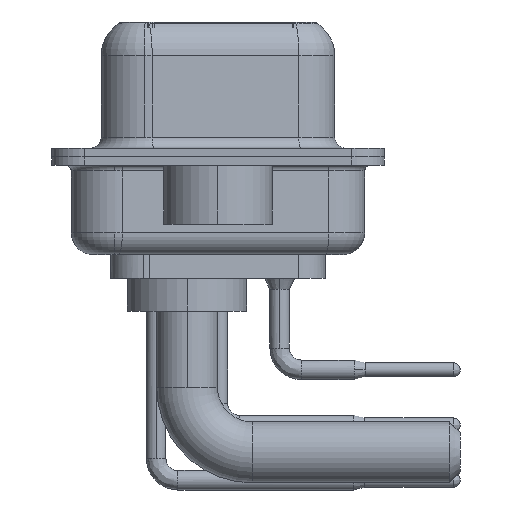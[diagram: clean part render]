
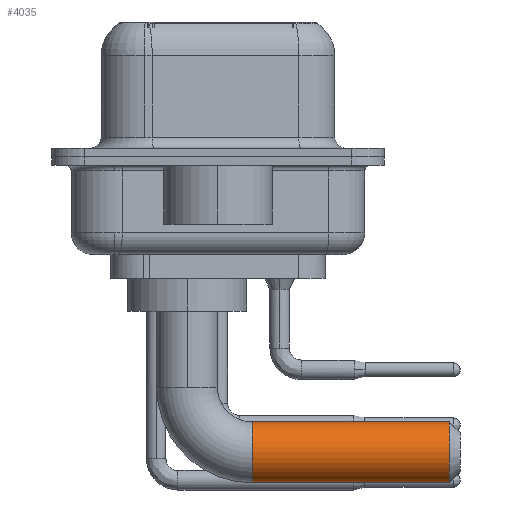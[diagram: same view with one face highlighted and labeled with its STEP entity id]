
A CAD part, left-side view. The second image highlights one B-rep face of the part: STEP entity #4035.
In plain terms, the highlighted cylindrical face has radius 1.4 mm (diameter 2.8 mm), a partial arc.
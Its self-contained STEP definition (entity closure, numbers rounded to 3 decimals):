
#2167 = CIRCLE ( 'NONE', #16886, 1.4 ) ;
#2221 = CARTESIAN_POINT ( 'NONE',  ( 0., -3., -5.1 ) ) ;
#2229 = CARTESIAN_POINT ( 'NONE',  ( 0., -3., -5.1 ) ) ;
#2546 = ORIENTED_EDGE ( 'NONE', *, *, #19837, .F. ) ;
#2560 = VECTOR ( 'NONE', #22478, 1000. ) ;
#2872 = CARTESIAN_POINT ( 'NONE',  ( 0., -3., -7.9 ) ) ;
#3657 = VERTEX_POINT ( 'NONE', #22633 ) ;
#4035 = ADVANCED_FACE ( 'NONE', ( #11558 ), #21620, .T. ) ;
#4675 = LINE ( 'NONE', #2221, #2560 ) ;
#5948 = VECTOR ( 'NONE', #7433, 1000. ) ;
#6181 = EDGE_CURVE ( 'NONE', #3657, #20578, #2167, .T. ) ;
#6552 = AXIS2_PLACEMENT_3D ( 'NONE', #9235, #21592, #16998 ) ;
#6628 = DIRECTION ( 'NONE',  ( 0., -1., 0. ) ) ;
#6960 = EDGE_LOOP ( 'NONE', ( #2546, #9460, #12795, #32420 ) ) ;
#7433 = DIRECTION ( 'NONE',  ( 0., -1., 0. ) ) ;
#9235 = CARTESIAN_POINT ( 'NONE',  ( 0., -3., -6.5 ) ) ;
#9460 = ORIENTED_EDGE ( 'NONE', *, *, #11799, .T. ) ;
#11300 = CIRCLE ( 'NONE', #6552, 1.4 ) ;
#11558 = FACE_OUTER_BOUND ( 'NONE', #6960, .T. ) ;
#11799 = EDGE_CURVE ( 'NONE', #23588, #30888, #11300, .T. ) ;
#12795 = ORIENTED_EDGE ( 'NONE', *, *, #26847, .T. ) ;
#13920 = AXIS2_PLACEMENT_3D ( 'NONE', #29219, #6628, #16688 ) ;
#16688 = DIRECTION ( 'NONE',  ( 0., 0., -1. ) ) ;
#16886 = AXIS2_PLACEMENT_3D ( 'NONE', #29506, #21588, #19141 ) ;
#16998 = DIRECTION ( 'NONE',  ( -1., 0., 0. ) ) ;
#19141 = DIRECTION ( 'NONE',  ( 0., 0., -1. ) ) ;
#19837 = EDGE_CURVE ( 'NONE', #23588, #20578, #4675, .T. ) ;
#20288 = LINE ( 'NONE', #24933, #5948 ) ;
#20578 = VERTEX_POINT ( 'NONE', #30408 ) ;
#21588 = DIRECTION ( 'NONE',  ( 0., 1., 0. ) ) ;
#21592 = DIRECTION ( 'NONE',  ( 0., -1., 0. ) ) ;
#21620 = CYLINDRICAL_SURFACE ( 'NONE', #13920, 1.4 ) ;
#22478 = DIRECTION ( 'NONE',  ( 0., -1., 0. ) ) ;
#22633 = CARTESIAN_POINT ( 'NONE',  ( 0., -12.07, -7.9 ) ) ;
#23588 = VERTEX_POINT ( 'NONE', #2229 ) ;
#24933 = CARTESIAN_POINT ( 'NONE',  ( 0., -3., -7.9 ) ) ;
#26847 = EDGE_CURVE ( 'NONE', #30888, #3657, #20288, .T. ) ;
#29219 = CARTESIAN_POINT ( 'NONE',  ( 0., -3., -6.5 ) ) ;
#29506 = CARTESIAN_POINT ( 'NONE',  ( 0., -12.07, -6.5 ) ) ;
#30408 = CARTESIAN_POINT ( 'NONE',  ( 0., -12.07, -5.1 ) ) ;
#30888 = VERTEX_POINT ( 'NONE', #2872 ) ;
#32420 = ORIENTED_EDGE ( 'NONE', *, *, #6181, .T. ) ;
